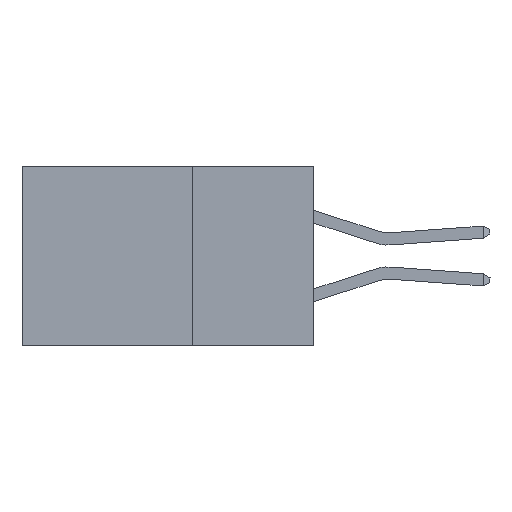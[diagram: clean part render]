
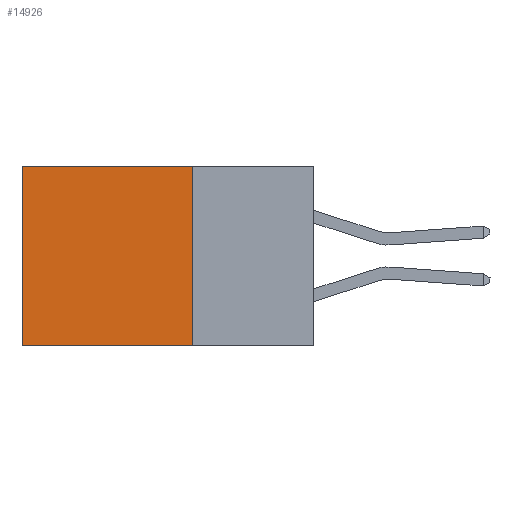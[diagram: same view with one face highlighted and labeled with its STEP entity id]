
A CAD part, left-side view. The second image highlights one B-rep face of the part: STEP entity #14926.
In plain terms, the highlighted planar face has unit normal (-1, 0, 0).
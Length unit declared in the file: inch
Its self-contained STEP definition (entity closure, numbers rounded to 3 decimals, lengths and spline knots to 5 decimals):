
#299 = CARTESIAN_POINT ( 'NONE',  ( 0.2875, 0.25, 0. ) ) ;
#2720 = VECTOR ( 'NONE', #30583, 39.37008 ) ;
#2828 = VERTEX_POINT ( 'NONE', #9784 ) ;
#3492 = EDGE_CURVE ( 'NONE', #32689, #23888, #24815, .T. ) ;
#4700 = LINE ( 'NONE', #37073, #2720 ) ;
#5492 = CARTESIAN_POINT ( 'NONE',  ( 0.2875, 0.25, 0. ) ) ;
#7063 = CARTESIAN_POINT ( 'NONE',  ( 0.2875, 0.25, 0. ) ) ;
#7377 = EDGE_CURVE ( 'NONE', #2828, #23888, #4700, .T. ) ;
#8018 = VECTOR ( 'NONE', #17018, 39.37008 ) ;
#9784 = CARTESIAN_POINT ( 'NONE',  ( 0.2875, 0.6, 0. ) ) ;
#10631 = ORIENTED_EDGE ( 'NONE', *, *, #25739, .T. ) ;
#12378 = PLANE ( 'NONE',  #31644 ) ;
#14379 = CARTESIAN_POINT ( 'NONE',  ( 0.2875, 0.25, -0.37 ) ) ;
#14926 = ADVANCED_FACE ( 'NONE', ( #32410 ), #12378, .F. ) ;
#14942 = VECTOR ( 'NONE', #39232, 39.37008 ) ;
#17018 = DIRECTION ( 'NONE',  ( 0., 1., 0. ) ) ;
#18089 = ORIENTED_EDGE ( 'NONE', *, *, #33188, .F. ) ;
#19160 = VECTOR ( 'NONE', #21201, 39.37008 ) ;
#21201 = DIRECTION ( 'NONE',  ( 0., 1., 0. ) ) ;
#21967 = DIRECTION ( 'NONE',  ( 0., 0., -1. ) ) ;
#22247 = DIRECTION ( 'NONE',  ( 1., 0., 0. ) ) ;
#23173 = LINE ( 'NONE', #29850, #14942 ) ;
#23888 = VERTEX_POINT ( 'NONE', #25987 ) ;
#24798 = CARTESIAN_POINT ( 'NONE',  ( 0.2875, 0.25, -0.37 ) ) ;
#24815 = LINE ( 'NONE', #14379, #8018 ) ;
#25739 = EDGE_CURVE ( 'NONE', #39129, #2828, #27546, .T. ) ;
#25987 = CARTESIAN_POINT ( 'NONE',  ( 0.2875, 0.6, -0.37 ) ) ;
#27546 = LINE ( 'NONE', #5492, #19160 ) ;
#29850 = CARTESIAN_POINT ( 'NONE',  ( 0.2875, 0.25, 0. ) ) ;
#30583 = DIRECTION ( 'NONE',  ( 0., 0., -1. ) ) ;
#31259 = ORIENTED_EDGE ( 'NONE', *, *, #7377, .T. ) ;
#31644 = AXIS2_PLACEMENT_3D ( 'NONE', #299, #22247, #21967 ) ;
#32410 = FACE_OUTER_BOUND ( 'NONE', #40392, .T. ) ;
#32689 = VERTEX_POINT ( 'NONE', #24798 ) ;
#33188 = EDGE_CURVE ( 'NONE', #39129, #32689, #23173, .T. ) ;
#35403 = ORIENTED_EDGE ( 'NONE', *, *, #3492, .F. ) ;
#37073 = CARTESIAN_POINT ( 'NONE',  ( 0.2875, 0.6, 0. ) ) ;
#39129 = VERTEX_POINT ( 'NONE', #7063 ) ;
#39232 = DIRECTION ( 'NONE',  ( 0., 0., -1. ) ) ;
#40392 = EDGE_LOOP ( 'NONE', ( #31259, #35403, #18089, #10631 ) ) ;
